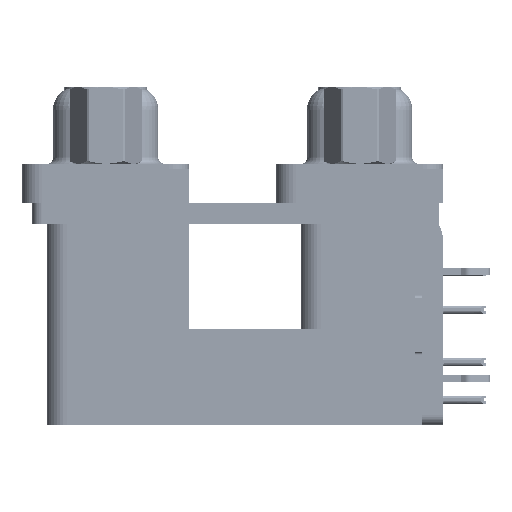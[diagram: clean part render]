
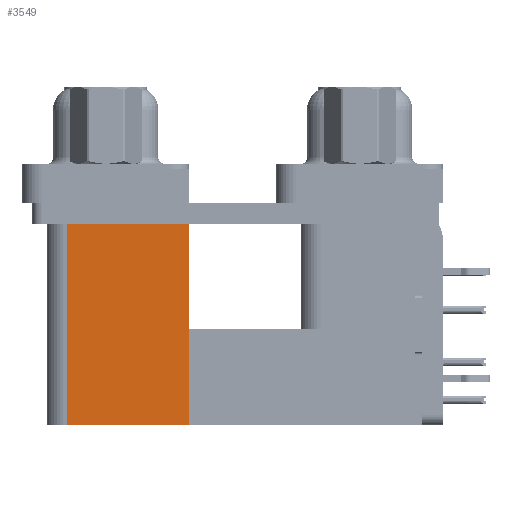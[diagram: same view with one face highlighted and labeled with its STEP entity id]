
A CAD part, left-side view. The second image highlights one B-rep face of the part: STEP entity #3549.
In plain terms, the highlighted planar face has unit normal (-1, 0, 0).
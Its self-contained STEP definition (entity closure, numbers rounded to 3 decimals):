
#471 = DIRECTION ( 'NONE',  ( 0., 0., 1. ) ) ;
#2999 = CARTESIAN_POINT ( 'NONE',  ( 3.765, 21.975, -19.2 ) ) ;
#3527 = ORIENTED_EDGE ( 'NONE', *, *, #38268, .T. ) ;
#3549 = ADVANCED_FACE ( 'NONE', ( #4937 ), #44796, .F. ) ;
#4937 = FACE_OUTER_BOUND ( 'NONE', #13218, .T. ) ;
#5792 = DIRECTION ( 'NONE',  ( 0., 0., -1. ) ) ;
#6821 = CARTESIAN_POINT ( 'NONE',  ( 3.765, 21.975, -19.2 ) ) ;
#7957 = VECTOR ( 'NONE', #21548, 1000. ) ;
#8185 = LINE ( 'NONE', #25802, #7957 ) ;
#8819 = EDGE_CURVE ( 'NONE', #31644, #46566, #16999, .T. ) ;
#13218 = EDGE_LOOP ( 'NONE', ( #19601, #19680, #49906, #3527 ) ) ;
#13614 = CARTESIAN_POINT ( 'NONE',  ( 3.765, 12.775, -19.2 ) ) ;
#16999 = LINE ( 'NONE', #56272, #20255 ) ;
#19438 = CARTESIAN_POINT ( 'NONE',  ( 3.765, 21.975, -2.5 ) ) ;
#19601 = ORIENTED_EDGE ( 'NONE', *, *, #8819, .T. ) ;
#19680 = ORIENTED_EDGE ( 'NONE', *, *, #54830, .F. ) ;
#20255 = VECTOR ( 'NONE', #42337, 1000. ) ;
#21548 = DIRECTION ( 'NONE',  ( 0., 1., 0. ) ) ;
#22714 = AXIS2_PLACEMENT_3D ( 'NONE', #48778, #52776, #5792 ) ;
#25802 = CARTESIAN_POINT ( 'NONE',  ( 3.765, 12.775, -19.2 ) ) ;
#29725 = LINE ( 'NONE', #2999, #42535 ) ;
#31435 = VERTEX_POINT ( 'NONE', #32359 ) ;
#31644 = VERTEX_POINT ( 'NONE', #41076 ) ;
#32359 = CARTESIAN_POINT ( 'NONE',  ( 3.765, 12.775, -19.2 ) ) ;
#38268 = EDGE_CURVE ( 'NONE', #31435, #31644, #44047, .T. ) ;
#40842 = VERTEX_POINT ( 'NONE', #6821 ) ;
#41076 = CARTESIAN_POINT ( 'NONE',  ( 3.765, 12.775, -2.5 ) ) ;
#42337 = DIRECTION ( 'NONE',  ( 0., 1., 0. ) ) ;
#42535 = VECTOR ( 'NONE', #50833, 1000. ) ;
#44047 = LINE ( 'NONE', #13614, #51667 ) ;
#44796 = PLANE ( 'NONE',  #22714 ) ;
#46566 = VERTEX_POINT ( 'NONE', #19438 ) ;
#48778 = CARTESIAN_POINT ( 'NONE',  ( 3.765, 12.775, -19.2 ) ) ;
#49906 = ORIENTED_EDGE ( 'NONE', *, *, #54433, .F. ) ;
#50833 = DIRECTION ( 'NONE',  ( 0., 0., 1. ) ) ;
#51667 = VECTOR ( 'NONE', #471, 1000. ) ;
#52776 = DIRECTION ( 'NONE',  ( 1., 0., 0. ) ) ;
#54433 = EDGE_CURVE ( 'NONE', #31435, #40842, #8185, .T. ) ;
#54830 = EDGE_CURVE ( 'NONE', #40842, #46566, #29725, .T. ) ;
#56272 = CARTESIAN_POINT ( 'NONE',  ( 3.765, 12.775, -2.5 ) ) ;
